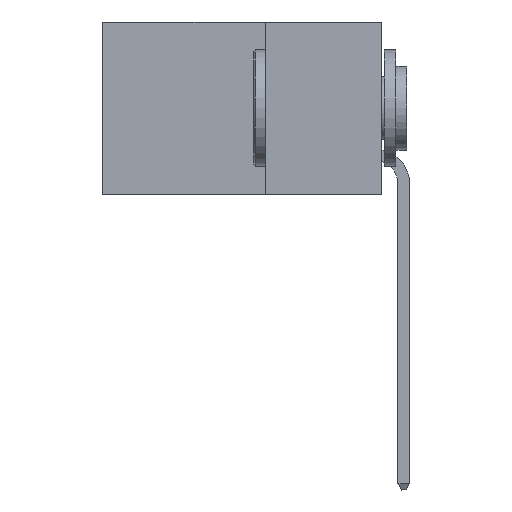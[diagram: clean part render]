
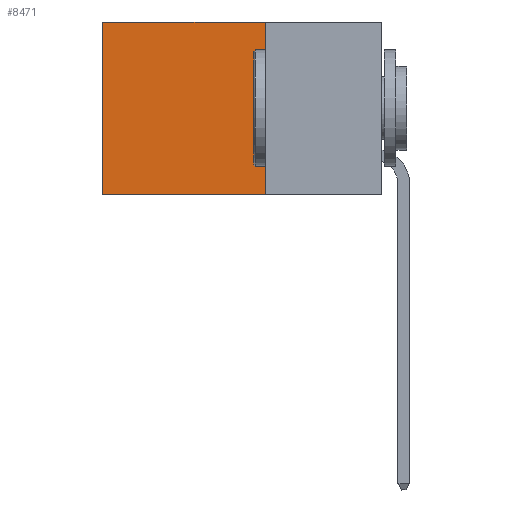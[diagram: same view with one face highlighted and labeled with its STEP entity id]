
A CAD part, left-side view. The second image highlights one B-rep face of the part: STEP entity #8471.
In plain terms, the highlighted planar face has unit normal (-1, 0, 0).
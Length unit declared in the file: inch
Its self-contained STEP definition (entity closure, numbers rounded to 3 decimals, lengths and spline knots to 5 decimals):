
#1400 = CARTESIAN_POINT ( 'NONE',  ( 0.2875, 0.6, 0. ) ) ;
#2158 = EDGE_CURVE ( 'NONE', #15168, #24213, #25184, .T. ) ;
#2384 = CARTESIAN_POINT ( 'NONE',  ( 0.2875, 0.25, -0.37 ) ) ;
#2979 = EDGE_CURVE ( 'NONE', #13076, #18220, #7245, .T. ) ;
#3595 = EDGE_CURVE ( 'NONE', #18220, #24213, #7186, .T. ) ;
#4544 = CARTESIAN_POINT ( 'NONE',  ( 0.2875, 0.25, 0. ) ) ;
#4549 = CARTESIAN_POINT ( 'NONE',  ( 0.2875, 0.25, 0. ) ) ;
#4952 = EDGE_LOOP ( 'NONE', ( #6916, #22604, #6345, #21089 ) ) ;
#5590 = DIRECTION ( 'NONE',  ( 0., 0., -1. ) ) ;
#6345 = ORIENTED_EDGE ( 'NONE', *, *, #2979, .F. ) ;
#6615 = CARTESIAN_POINT ( 'NONE',  ( 0.2875, 0.6, -0.37 ) ) ;
#6916 = ORIENTED_EDGE ( 'NONE', *, *, #2158, .T. ) ;
#7099 = LINE ( 'NONE', #4549, #27057 ) ;
#7186 = LINE ( 'NONE', #9957, #11940 ) ;
#7245 = LINE ( 'NONE', #4544, #27864 ) ;
#7957 = DIRECTION ( 'NONE',  ( 0., 1., 0. ) ) ;
#8246 = CARTESIAN_POINT ( 'NONE',  ( 0.2875, 0.25, 0. ) ) ;
#8471 = ADVANCED_FACE ( 'NONE', ( #23254 ), #14588, .F. ) ;
#9063 = DIRECTION ( 'NONE',  ( 0., 0., -1. ) ) ;
#9957 = CARTESIAN_POINT ( 'NONE',  ( 0.2875, 0.25, -0.37 ) ) ;
#10133 = CARTESIAN_POINT ( 'NONE',  ( 0.2875, 0.6, 0. ) ) ;
#11381 = CARTESIAN_POINT ( 'NONE',  ( 0.2875, 0.25, 0. ) ) ;
#11426 = AXIS2_PLACEMENT_3D ( 'NONE', #11381, #14466, #9063 ) ;
#11940 = VECTOR ( 'NONE', #7957, 39.37008 ) ;
#13076 = VERTEX_POINT ( 'NONE', #8246 ) ;
#13993 = EDGE_CURVE ( 'NONE', #13076, #15168, #7099, .T. ) ;
#14182 = DIRECTION ( 'NONE',  ( 0., 0., -1. ) ) ;
#14466 = DIRECTION ( 'NONE',  ( 1., 0., 0. ) ) ;
#14588 = PLANE ( 'NONE',  #11426 ) ;
#15168 = VERTEX_POINT ( 'NONE', #1400 ) ;
#18220 = VERTEX_POINT ( 'NONE', #2384 ) ;
#21089 = ORIENTED_EDGE ( 'NONE', *, *, #13993, .T. ) ;
#22105 = VECTOR ( 'NONE', #5590, 39.37008 ) ;
#22604 = ORIENTED_EDGE ( 'NONE', *, *, #3595, .F. ) ;
#23254 = FACE_OUTER_BOUND ( 'NONE', #4952, .T. ) ;
#24213 = VERTEX_POINT ( 'NONE', #6615 ) ;
#25184 = LINE ( 'NONE', #10133, #22105 ) ;
#26188 = DIRECTION ( 'NONE',  ( 0., 1., 0. ) ) ;
#27057 = VECTOR ( 'NONE', #26188, 39.37008 ) ;
#27864 = VECTOR ( 'NONE', #14182, 39.37008 ) ;
